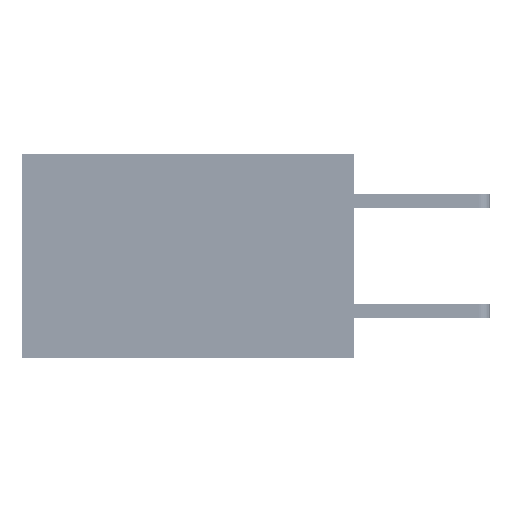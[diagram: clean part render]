
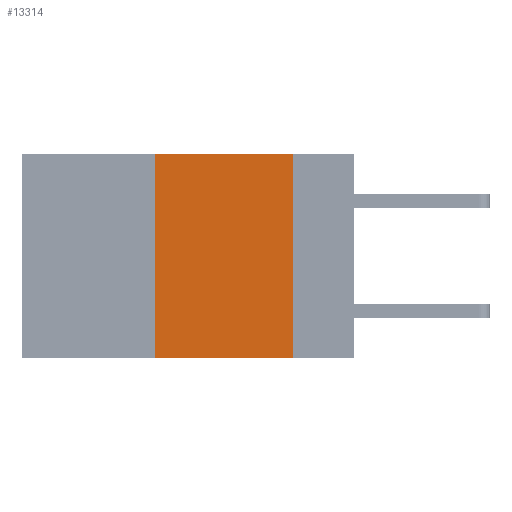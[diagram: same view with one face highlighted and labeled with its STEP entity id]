
A CAD part, left-side view. The second image highlights one B-rep face of the part: STEP entity #13314.
In plain terms, the highlighted planar face has unit normal (-1, 0, 0).
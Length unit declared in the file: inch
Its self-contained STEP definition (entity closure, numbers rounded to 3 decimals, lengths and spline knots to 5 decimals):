
#57 = VERTEX_POINT ( 'NONE', #16381 ) ;
#2653 = CARTESIAN_POINT ( 'NONE',  ( 0., 0.36, 0. ) ) ;
#3412 = DIRECTION ( 'NONE',  ( 0., 0., -1. ) ) ;
#3815 = LINE ( 'NONE', #40625, #31401 ) ;
#5659 = CARTESIAN_POINT ( 'NONE',  ( 0., 0.11, -0.37 ) ) ;
#5733 = DIRECTION ( 'NONE',  ( 0., 0., -1. ) ) ;
#8028 = ORIENTED_EDGE ( 'NONE', *, *, #17563, .F. ) ;
#9597 = CARTESIAN_POINT ( 'NONE',  ( 0., 0.11, 0. ) ) ;
#10157 = ORIENTED_EDGE ( 'NONE', *, *, #15244, .T. ) ;
#13314 = ADVANCED_FACE ( 'NONE', ( #37374 ), #43654, .F. ) ;
#13900 = VECTOR ( 'NONE', #3412, 39.37008 ) ;
#14994 = LINE ( 'NONE', #9597, #13900 ) ;
#15244 = EDGE_CURVE ( 'NONE', #57, #35968, #33775, .T. ) ;
#16238 = DIRECTION ( 'NONE',  ( 0., -1., 0. ) ) ;
#16381 = CARTESIAN_POINT ( 'NONE',  ( 0., 0.36, -0.37 ) ) ;
#16493 = VECTOR ( 'NONE', #34636, 39.37008 ) ;
#17254 = CARTESIAN_POINT ( 'NONE',  ( 0., 0.11, 0. ) ) ;
#17563 = EDGE_CURVE ( 'NONE', #57, #37665, #3815, .T. ) ;
#20109 = VERTEX_POINT ( 'NONE', #17254 ) ;
#23037 = CARTESIAN_POINT ( 'NONE',  ( 0., 0.6, 0. ) ) ;
#26450 = DIRECTION ( 'NONE',  ( 1., 0., 0. ) ) ;
#29063 = EDGE_CURVE ( 'NONE', #20109, #35968, #14994, .T. ) ;
#30410 = DIRECTION ( 'NONE',  ( 0., 0., 1. ) ) ;
#31044 = EDGE_CURVE ( 'NONE', #37665, #20109, #35808, .T. ) ;
#31205 = CARTESIAN_POINT ( 'NONE',  ( 0., 0.6, 0. ) ) ;
#31236 = ORIENTED_EDGE ( 'NONE', *, *, #29063, .F. ) ;
#31401 = VECTOR ( 'NONE', #30410, 39.37008 ) ;
#31771 = ORIENTED_EDGE ( 'NONE', *, *, #31044, .F. ) ;
#33775 = LINE ( 'NONE', #40263, #42983 ) ;
#34636 = DIRECTION ( 'NONE',  ( 0., -1., 0. ) ) ;
#35808 = LINE ( 'NONE', #31205, #16493 ) ;
#35968 = VERTEX_POINT ( 'NONE', #5659 ) ;
#37374 = FACE_OUTER_BOUND ( 'NONE', #40463, .T. ) ;
#37665 = VERTEX_POINT ( 'NONE', #2653 ) ;
#40263 = CARTESIAN_POINT ( 'NONE',  ( 0., 0.6, -0.37 ) ) ;
#40463 = EDGE_LOOP ( 'NONE', ( #31236, #31771, #8028, #10157 ) ) ;
#40625 = CARTESIAN_POINT ( 'NONE',  ( 0., 0.36, 0. ) ) ;
#42983 = VECTOR ( 'NONE', #16238, 39.37008 ) ;
#43654 = PLANE ( 'NONE',  #44323 ) ;
#44323 = AXIS2_PLACEMENT_3D ( 'NONE', #23037, #26450, #5733 ) ;
